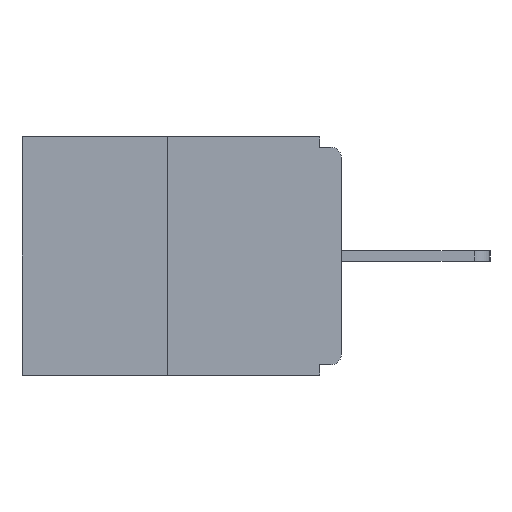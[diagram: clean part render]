
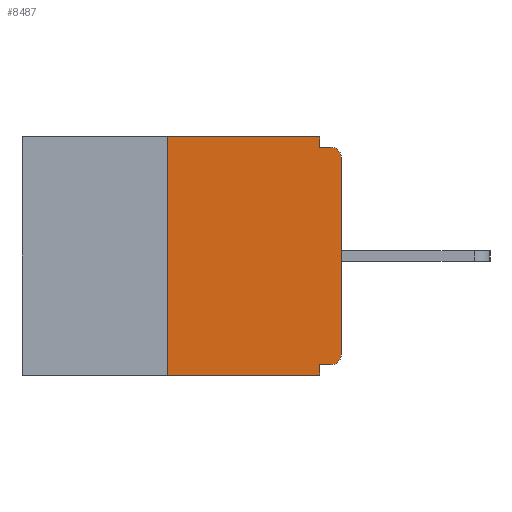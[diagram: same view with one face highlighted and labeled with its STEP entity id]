
A CAD part, left-side view. The second image highlights one B-rep face of the part: STEP entity #8487.
In plain terms, the highlighted planar face has unit normal (-1, 0, 0).
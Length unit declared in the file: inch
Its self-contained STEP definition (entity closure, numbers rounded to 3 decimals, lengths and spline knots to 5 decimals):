
#645 = CARTESIAN_POINT ( 'NONE',  ( 0., 0.015, -0.313 ) ) ;
#971 = CARTESIAN_POINT ( 'NONE',  ( 0., 0.015, -0.015 ) ) ;
#1090 = EDGE_CURVE ( 'NONE', #5953, #9632, #13962, .T. ) ;
#1226 = VERTEX_POINT ( 'NONE', #1938 ) ;
#1379 = DIRECTION ( 'NONE',  ( 0., 0., -1. ) ) ;
#1568 = DIRECTION ( 'NONE',  ( 0., 0., -1. ) ) ;
#1650 = CIRCLE ( 'NONE', #2824, 0.015 ) ;
#1687 = DIRECTION ( 'NONE',  ( 0., 0., -1. ) ) ;
#1903 = ORIENTED_EDGE ( 'NONE', *, *, #8781, .F. ) ;
#1938 = CARTESIAN_POINT ( 'NONE',  ( 0., 0.015, -0.328 ) ) ;
#2000 = ORIENTED_EDGE ( 'NONE', *, *, #14550, .F. ) ;
#2106 = LINE ( 'NONE', #2242, #12759 ) ;
#2230 = ORIENTED_EDGE ( 'NONE', *, *, #8708, .T. ) ;
#2242 = CARTESIAN_POINT ( 'NONE',  ( 0., 0., -0.328 ) ) ;
#2347 = VECTOR ( 'NONE', #7588, 39.37008 ) ;
#2393 = CARTESIAN_POINT ( 'NONE',  ( 0., 0., 0. ) ) ;
#2557 = CARTESIAN_POINT ( 'NONE',  ( 0., 0., -0.03 ) ) ;
#2824 = AXIS2_PLACEMENT_3D ( 'NONE', #645, #13033, #7613 ) ;
#2826 = CARTESIAN_POINT ( 'NONE',  ( 0., 0.031, 0. ) ) ;
#2907 = ORIENTED_EDGE ( 'NONE', *, *, #4508, .F. ) ;
#3144 = ORIENTED_EDGE ( 'NONE', *, *, #8824, .T. ) ;
#3387 = DIRECTION ( 'NONE',  ( 0., 0., 1. ) ) ;
#3580 = FACE_OUTER_BOUND ( 'NONE', #7667, .T. ) ;
#3600 = VERTEX_POINT ( 'NONE', #2826 ) ;
#3706 = CARTESIAN_POINT ( 'NONE',  ( 0., 0., -0.015 ) ) ;
#3736 = VECTOR ( 'NONE', #10082, 39.37008 ) ;
#3772 = CARTESIAN_POINT ( 'NONE',  ( 0., 0.031, -0.343 ) ) ;
#4158 = VECTOR ( 'NONE', #13439, 39.37008 ) ;
#4302 = DIRECTION ( 'NONE',  ( 0., 1., 0. ) ) ;
#4373 = LINE ( 'NONE', #2393, #3736 ) ;
#4503 = CARTESIAN_POINT ( 'NONE',  ( 0., 0.46, 0. ) ) ;
#4508 = EDGE_CURVE ( 'NONE', #3600, #6387, #7394, .T. ) ;
#4813 = VERTEX_POINT ( 'NONE', #10185 ) ;
#4931 = VECTOR ( 'NONE', #8254, 39.37008 ) ;
#5206 = CARTESIAN_POINT ( 'NONE',  ( 0., 0.25, -0.343 ) ) ;
#5253 = CARTESIAN_POINT ( 'NONE',  ( 0., 0.46, -0.343 ) ) ;
#5313 = ORIENTED_EDGE ( 'NONE', *, *, #6139, .F. ) ;
#5379 = EDGE_CURVE ( 'NONE', #6387, #13240, #12789, .T. ) ;
#5509 = EDGE_CURVE ( 'NONE', #12276, #9632, #7859, .T. ) ;
#5834 = LINE ( 'NONE', #6813, #10067 ) ;
#5953 = VERTEX_POINT ( 'NONE', #8324 ) ;
#5998 = CARTESIAN_POINT ( 'NONE',  ( 0., 0.015, -0.03 ) ) ;
#6139 = EDGE_CURVE ( 'NONE', #12276, #4813, #5834, .T. ) ;
#6387 = VERTEX_POINT ( 'NONE', #13860 ) ;
#6788 = VECTOR ( 'NONE', #8307, 39.37008 ) ;
#6813 = CARTESIAN_POINT ( 'NONE',  ( 0., 0.25, 0. ) ) ;
#7394 = LINE ( 'NONE', #10490, #10220 ) ;
#7549 = AXIS2_PLACEMENT_3D ( 'NONE', #11522, #9356, #1379 ) ;
#7588 = DIRECTION ( 'NONE',  ( 0., -1., 0. ) ) ;
#7613 = DIRECTION ( 'NONE',  ( 0., 0., -1. ) ) ;
#7667 = EDGE_LOOP ( 'NONE', ( #2000, #5313, #9602, #9555, #1903, #11500, #2230, #3144, #10269, #2907 ) ) ;
#7859 = LINE ( 'NONE', #5253, #2347 ) ;
#8254 = DIRECTION ( 'NONE',  ( 0., -1., 0. ) ) ;
#8307 = DIRECTION ( 'NONE',  ( 0., 0., -1. ) ) ;
#8324 = CARTESIAN_POINT ( 'NONE',  ( 0., 0.031, -0.328 ) ) ;
#8487 = ADVANCED_FACE ( 'NONE', ( #3580 ), #12644, .F. ) ;
#8708 = EDGE_CURVE ( 'NONE', #13574, #12091, #4373, .T. ) ;
#8781 = EDGE_CURVE ( 'NONE', #1226, #5953, #2106, .T. ) ;
#8824 = EDGE_CURVE ( 'NONE', #12091, #13240, #9895, .T. ) ;
#8880 = CARTESIAN_POINT ( 'NONE',  ( 0., 0.031, -0.343 ) ) ;
#9356 = DIRECTION ( 'NONE',  ( 1., 0., 0. ) ) ;
#9555 = ORIENTED_EDGE ( 'NONE', *, *, #1090, .F. ) ;
#9602 = ORIENTED_EDGE ( 'NONE', *, *, #5509, .T. ) ;
#9632 = VERTEX_POINT ( 'NONE', #8880 ) ;
#9895 = CIRCLE ( 'NONE', #11815, 0.015 ) ;
#10061 = LINE ( 'NONE', #4503, #4158 ) ;
#10067 = VECTOR ( 'NONE', #3387, 39.37008 ) ;
#10082 = DIRECTION ( 'NONE',  ( 0., 0., 1. ) ) ;
#10185 = CARTESIAN_POINT ( 'NONE',  ( 0., 0.25, 0. ) ) ;
#10220 = VECTOR ( 'NONE', #1687, 39.37008 ) ;
#10269 = ORIENTED_EDGE ( 'NONE', *, *, #5379, .F. ) ;
#10490 = CARTESIAN_POINT ( 'NONE',  ( 0., 0.031, 0. ) ) ;
#10719 = EDGE_CURVE ( 'NONE', #1226, #13574, #1650, .T. ) ;
#11500 = ORIENTED_EDGE ( 'NONE', *, *, #10719, .T. ) ;
#11522 = CARTESIAN_POINT ( 'NONE',  ( 0., 0.46, 0. ) ) ;
#11723 = DIRECTION ( 'NONE',  ( -1., 0., 0. ) ) ;
#11771 = CARTESIAN_POINT ( 'NONE',  ( 0., 0., -0.313 ) ) ;
#11815 = AXIS2_PLACEMENT_3D ( 'NONE', #5998, #11723, #1568 ) ;
#12091 = VERTEX_POINT ( 'NONE', #2557 ) ;
#12276 = VERTEX_POINT ( 'NONE', #5206 ) ;
#12644 = PLANE ( 'NONE',  #7549 ) ;
#12759 = VECTOR ( 'NONE', #4302, 39.37008 ) ;
#12789 = LINE ( 'NONE', #3706, #4931 ) ;
#13033 = DIRECTION ( 'NONE',  ( -1., 0., 0. ) ) ;
#13240 = VERTEX_POINT ( 'NONE', #971 ) ;
#13439 = DIRECTION ( 'NONE',  ( 0., -1., 0. ) ) ;
#13574 = VERTEX_POINT ( 'NONE', #11771 ) ;
#13860 = CARTESIAN_POINT ( 'NONE',  ( 0., 0.031, -0.015 ) ) ;
#13962 = LINE ( 'NONE', #3772, #6788 ) ;
#14550 = EDGE_CURVE ( 'NONE', #4813, #3600, #10061, .T. ) ;
